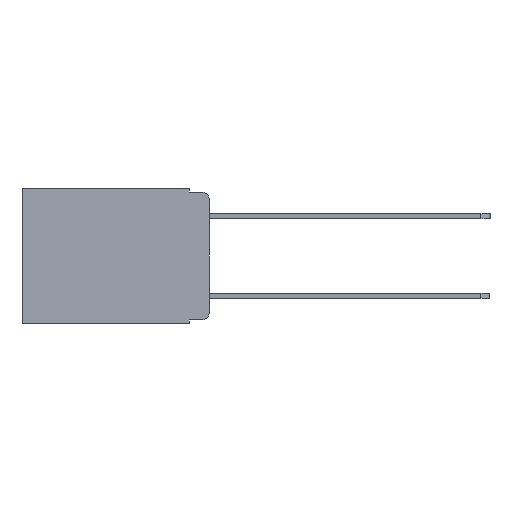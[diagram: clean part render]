
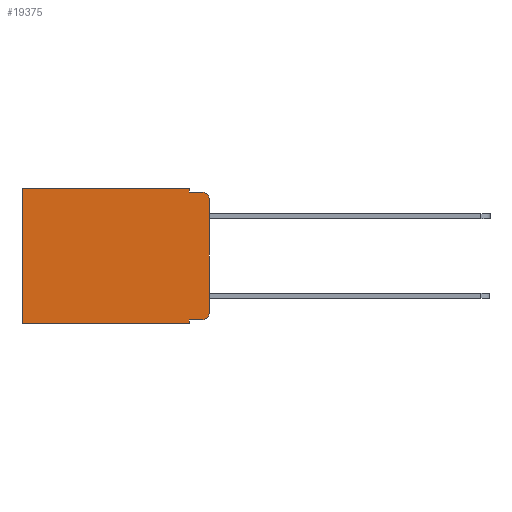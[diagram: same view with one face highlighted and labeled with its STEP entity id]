
A CAD part, left-side view. The second image highlights one B-rep face of the part: STEP entity #19375.
In plain terms, the highlighted planar face has unit normal (-1, 0, 0).
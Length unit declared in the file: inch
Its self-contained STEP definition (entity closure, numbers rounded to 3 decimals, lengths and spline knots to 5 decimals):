
#16 = EDGE_CURVE ( 'NONE', #2213, #5039, #9519, .T. ) ;
#225 = VERTEX_POINT ( 'NONE', #6205 ) ;
#1090 = EDGE_CURVE ( 'NONE', #17188, #16468, #20540, .T. ) ;
#1140 = DIRECTION ( 'NONE',  ( 0., -1., 0. ) ) ;
#1220 = CARTESIAN_POINT ( 'NONE',  ( 0.298, 0.051, 0. ) ) ;
#1363 = DIRECTION ( 'NONE',  ( 1., 0., 0. ) ) ;
#1389 = DIRECTION ( 'NONE',  ( 0., 0., -1. ) ) ;
#2023 = CARTESIAN_POINT ( 'NONE',  ( 0.298, 0.02, -0.03 ) ) ;
#2213 = VERTEX_POINT ( 'NONE', #19396 ) ;
#2772 = ORIENTED_EDGE ( 'NONE', *, *, #13061, .F. ) ;
#2939 = ORIENTED_EDGE ( 'NONE', *, *, #6891, .T. ) ;
#3008 = VECTOR ( 'NONE', #13641, 39.37008 ) ;
#3339 = ORIENTED_EDGE ( 'NONE', *, *, #5650, .F. ) ;
#3525 = VERTEX_POINT ( 'NONE', #8957 ) ;
#3849 = DIRECTION ( 'NONE',  ( 0., 0., -1. ) ) ;
#4093 = FACE_OUTER_BOUND ( 'NONE', #11959, .T. ) ;
#4271 = CARTESIAN_POINT ( 'NONE',  ( 0.298, 0.051, -0.01 ) ) ;
#4446 = DIRECTION ( 'NONE',  ( 0., 1., 0. ) ) ;
#4783 = CARTESIAN_POINT ( 'NONE',  ( 0.298, 0.051, -0.01 ) ) ;
#4864 = EDGE_CURVE ( 'NONE', #13927, #2213, #15071, .T. ) ;
#5039 = VERTEX_POINT ( 'NONE', #13146 ) ;
#5086 = DIRECTION ( 'NONE',  ( 0., 0., -1. ) ) ;
#5455 = CARTESIAN_POINT ( 'NONE',  ( 0.298, 0.473, 0. ) ) ;
#5631 = AXIS2_PLACEMENT_3D ( 'NONE', #2023, #14568, #3849 ) ;
#5650 = EDGE_CURVE ( 'NONE', #225, #3525, #8423, .T. ) ;
#5745 = ORIENTED_EDGE ( 'NONE', *, *, #15597, .T. ) ;
#5907 = DIRECTION ( 'NONE',  ( -1., 0., 0. ) ) ;
#6140 = CIRCLE ( 'NONE', #18163, 0.02 ) ;
#6205 = CARTESIAN_POINT ( 'NONE',  ( 0.298, 0., -0.03 ) ) ;
#6697 = DIRECTION ( 'NONE',  ( 0., 0., -1. ) ) ;
#6891 = EDGE_CURVE ( 'NONE', #13624, #3525, #6140, .T. ) ;
#7838 = EDGE_CURVE ( 'NONE', #13927, #13624, #16590, .T. ) ;
#8423 = LINE ( 'NONE', #10157, #17150 ) ;
#8709 = VECTOR ( 'NONE', #5086, 39.37008 ) ;
#8957 = CARTESIAN_POINT ( 'NONE',  ( 0.298, 0., -0.313 ) ) ;
#9218 = DIRECTION ( 'NONE',  ( 0., 0., -1. ) ) ;
#9276 = LINE ( 'NONE', #20810, #8709 ) ;
#9519 = LINE ( 'NONE', #19881, #22696 ) ;
#9774 = ORIENTED_EDGE ( 'NONE', *, *, #1090, .F. ) ;
#10029 = CARTESIAN_POINT ( 'NONE',  ( 0.298, 0.02, -0.333 ) ) ;
#10157 = CARTESIAN_POINT ( 'NONE',  ( 0.298, 0., 0. ) ) ;
#10418 = PLANE ( 'NONE',  #13906 ) ;
#10470 = LINE ( 'NONE', #15058, #14547 ) ;
#11422 = VECTOR ( 'NONE', #1389, 39.37008 ) ;
#11959 = EDGE_LOOP ( 'NONE', ( #3339, #22180, #2772, #9774, #22400, #5745, #20295, #12253, #21881, #2939 ) ) ;
#12253 = ORIENTED_EDGE ( 'NONE', *, *, #4864, .F. ) ;
#13061 = EDGE_CURVE ( 'NONE', #16468, #16045, #20188, .T. ) ;
#13146 = CARTESIAN_POINT ( 'NONE',  ( 0.298, 0.473, -0.343 ) ) ;
#13571 = EDGE_CURVE ( 'NONE', #17188, #16252, #10470, .T. ) ;
#13624 = VERTEX_POINT ( 'NONE', #10029 ) ;
#13641 = DIRECTION ( 'NONE',  ( 0., -1., 0. ) ) ;
#13906 = AXIS2_PLACEMENT_3D ( 'NONE', #22406, #1363, #13936 ) ;
#13927 = VERTEX_POINT ( 'NONE', #17781 ) ;
#13936 = DIRECTION ( 'NONE',  ( 0., 0., -1. ) ) ;
#14547 = VECTOR ( 'NONE', #4446, 39.37008 ) ;
#14568 = DIRECTION ( 'NONE',  ( -1., 0., 0. ) ) ;
#15058 = CARTESIAN_POINT ( 'NONE',  ( 0.298, 0., 0. ) ) ;
#15071 = LINE ( 'NONE', #1220, #19087 ) ;
#15302 = CARTESIAN_POINT ( 'NONE',  ( 0.298, 0.051, 0. ) ) ;
#15597 = EDGE_CURVE ( 'NONE', #16252, #5039, #9276, .T. ) ;
#15645 = VECTOR ( 'NONE', #1140, 39.37008 ) ;
#15998 = CARTESIAN_POINT ( 'NONE',  ( 0.298, 0.051, 0. ) ) ;
#16045 = VERTEX_POINT ( 'NONE', #18865 ) ;
#16252 = VERTEX_POINT ( 'NONE', #5455 ) ;
#16468 = VERTEX_POINT ( 'NONE', #4271 ) ;
#16490 = CARTESIAN_POINT ( 'NONE',  ( 0.298, 0.02, -0.313 ) ) ;
#16590 = LINE ( 'NONE', #18870, #3008 ) ;
#17150 = VECTOR ( 'NONE', #9218, 39.37008 ) ;
#17188 = VERTEX_POINT ( 'NONE', #15302 ) ;
#17781 = CARTESIAN_POINT ( 'NONE',  ( 0.298, 0.051, -0.333 ) ) ;
#18163 = AXIS2_PLACEMENT_3D ( 'NONE', #16490, #5907, #18219 ) ;
#18219 = DIRECTION ( 'NONE',  ( 0., 0., -1. ) ) ;
#18323 = EDGE_CURVE ( 'NONE', #225, #16045, #21674, .T. ) ;
#18865 = CARTESIAN_POINT ( 'NONE',  ( 0.298, 0.02, -0.01 ) ) ;
#18870 = CARTESIAN_POINT ( 'NONE',  ( 0.298, 0.051, -0.333 ) ) ;
#19087 = VECTOR ( 'NONE', #6697, 39.37008 ) ;
#19375 = ADVANCED_FACE ( 'NONE', ( #4093 ), #10418, .F. ) ;
#19396 = CARTESIAN_POINT ( 'NONE',  ( 0.298, 0.051, -0.343 ) ) ;
#19881 = CARTESIAN_POINT ( 'NONE',  ( 0.298, 0., -0.343 ) ) ;
#20001 = DIRECTION ( 'NONE',  ( 0., 1., 0. ) ) ;
#20188 = LINE ( 'NONE', #4783, #15645 ) ;
#20295 = ORIENTED_EDGE ( 'NONE', *, *, #16, .F. ) ;
#20540 = LINE ( 'NONE', #15998, #11422 ) ;
#20810 = CARTESIAN_POINT ( 'NONE',  ( 0.298, 0.473, 0. ) ) ;
#21674 = CIRCLE ( 'NONE', #5631, 0.02 ) ;
#21881 = ORIENTED_EDGE ( 'NONE', *, *, #7838, .T. ) ;
#22180 = ORIENTED_EDGE ( 'NONE', *, *, #18323, .T. ) ;
#22400 = ORIENTED_EDGE ( 'NONE', *, *, #13571, .T. ) ;
#22406 = CARTESIAN_POINT ( 'NONE',  ( 0.298, 0., 0. ) ) ;
#22696 = VECTOR ( 'NONE', #20001, 39.37008 ) ;
